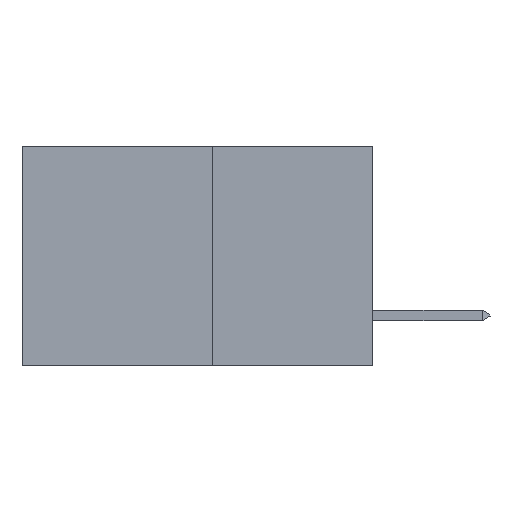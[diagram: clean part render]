
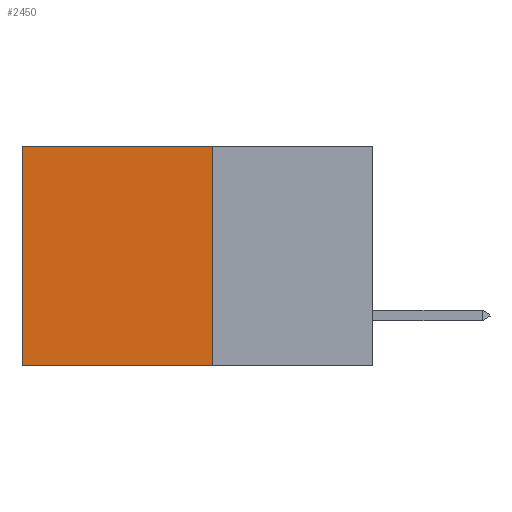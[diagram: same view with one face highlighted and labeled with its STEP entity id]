
A CAD part, left-side view. The second image highlights one B-rep face of the part: STEP entity #2450.
In plain terms, the highlighted planar face has unit normal (-1, 0, 0).
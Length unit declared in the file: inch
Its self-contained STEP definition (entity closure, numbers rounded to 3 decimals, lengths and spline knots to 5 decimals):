
#227 = VECTOR ( 'NONE', #4687, 39.37008 ) ;
#396 = AXIS2_PLACEMENT_3D ( 'NONE', #3536, #15462, #4903 ) ;
#401 = ORIENTED_EDGE ( 'NONE', *, *, #6425, .F. ) ;
#616 = VECTOR ( 'NONE', #12614, 39.37008 ) ;
#2450 = ADVANCED_FACE ( 'NONE', ( #20604 ), #8593, .F. ) ;
#2909 = VECTOR ( 'NONE', #4645, 39.37008 ) ;
#3287 = ORIENTED_EDGE ( 'NONE', *, *, #3726, .T. ) ;
#3536 = CARTESIAN_POINT ( 'NONE',  ( 0.277, 0.27, -0.37 ) ) ;
#3726 = EDGE_CURVE ( 'NONE', #14875, #15010, #10803, .T. ) ;
#3857 = CARTESIAN_POINT ( 'NONE',  ( 0.277, 0.59, -0.37 ) ) ;
#4645 = DIRECTION ( 'NONE',  ( 0., 1., 0. ) ) ;
#4687 = DIRECTION ( 'NONE',  ( 0., 0., -1. ) ) ;
#4903 = DIRECTION ( 'NONE',  ( 0., 0., -1. ) ) ;
#5410 = ORIENTED_EDGE ( 'NONE', *, *, #16843, .F. ) ;
#5990 = CARTESIAN_POINT ( 'NONE',  ( 0.277, 0.27, 0. ) ) ;
#6425 = EDGE_CURVE ( 'NONE', #7849, #15010, #9755, .T. ) ;
#7440 = DIRECTION ( 'NONE',  ( 0., 0., -1. ) ) ;
#7849 = VERTEX_POINT ( 'NONE', #21067 ) ;
#8593 = PLANE ( 'NONE',  #396 ) ;
#9001 = CARTESIAN_POINT ( 'NONE',  ( 0.277, 0.59, -0.37 ) ) ;
#9755 = LINE ( 'NONE', #12691, #616 ) ;
#10803 = LINE ( 'NONE', #3857, #16092 ) ;
#11780 = ORIENTED_EDGE ( 'NONE', *, *, #22080, .T. ) ;
#12213 = LINE ( 'NONE', #18656, #2909 ) ;
#12237 = EDGE_LOOP ( 'NONE', ( #3287, #401, #5410, #11780 ) ) ;
#12614 = DIRECTION ( 'NONE',  ( 0., 1., 0. ) ) ;
#12691 = CARTESIAN_POINT ( 'NONE',  ( 0.277, 0.27, -0.37 ) ) ;
#14875 = VERTEX_POINT ( 'NONE', #20469 ) ;
#15010 = VERTEX_POINT ( 'NONE', #9001 ) ;
#15462 = DIRECTION ( 'NONE',  ( 1., 0., 0. ) ) ;
#16092 = VECTOR ( 'NONE', #7440, 39.37008 ) ;
#16843 = EDGE_CURVE ( 'NONE', #17868, #7849, #22062, .T. ) ;
#16986 = CARTESIAN_POINT ( 'NONE',  ( 0.277, 0.27, -0.37 ) ) ;
#17868 = VERTEX_POINT ( 'NONE', #5990 ) ;
#18656 = CARTESIAN_POINT ( 'NONE',  ( 0.277, 0.27, 0. ) ) ;
#20469 = CARTESIAN_POINT ( 'NONE',  ( 0.277, 0.59, 0. ) ) ;
#20604 = FACE_OUTER_BOUND ( 'NONE', #12237, .T. ) ;
#21067 = CARTESIAN_POINT ( 'NONE',  ( 0.277, 0.27, -0.37 ) ) ;
#22062 = LINE ( 'NONE', #16986, #227 ) ;
#22080 = EDGE_CURVE ( 'NONE', #17868, #14875, #12213, .T. ) ;
